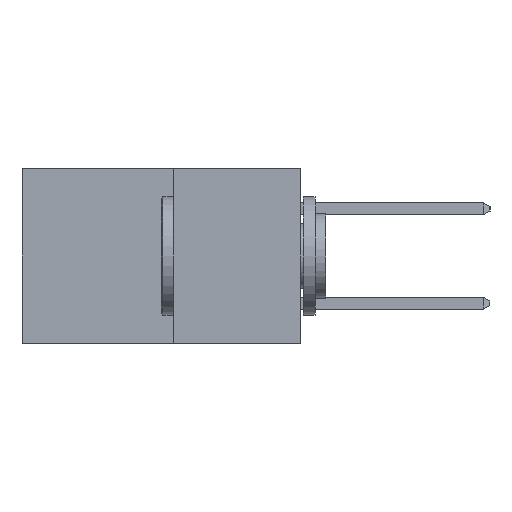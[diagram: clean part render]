
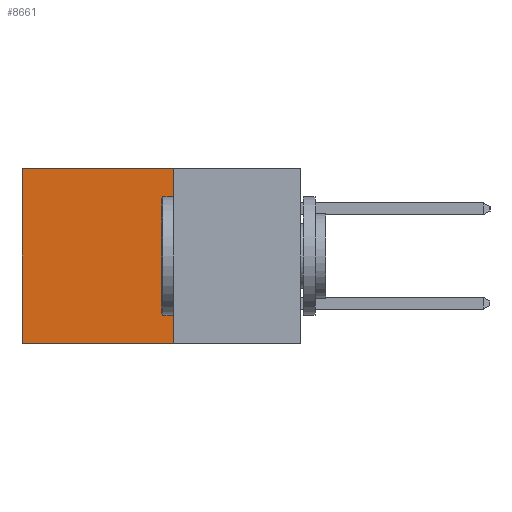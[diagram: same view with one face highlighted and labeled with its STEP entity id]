
A CAD part, left-side view. The second image highlights one B-rep face of the part: STEP entity #8661.
In plain terms, the highlighted planar face has unit normal (-1, 0, 0).
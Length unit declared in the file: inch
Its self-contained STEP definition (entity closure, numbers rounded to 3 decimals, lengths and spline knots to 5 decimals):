
#119 = CARTESIAN_POINT ( 'NONE',  ( 0.277, 0.59, -0.37 ) ) ;
#309 = LINE ( 'NONE', #3089, #3862 ) ;
#445 = LINE ( 'NONE', #697, #2233 ) ;
#697 = CARTESIAN_POINT ( 'NONE',  ( 0.277, 0.27, -0.37 ) ) ;
#1018 = EDGE_CURVE ( 'NONE', #4037, #9228, #309, .T. ) ;
#1445 = VECTOR ( 'NONE', #2529, 39.37008 ) ;
#1720 = CARTESIAN_POINT ( 'NONE',  ( 0.277, 0.27, 0. ) ) ;
#2233 = VECTOR ( 'NONE', #6638, 39.37008 ) ;
#2307 = EDGE_CURVE ( 'NONE', #4507, #9004, #8526, .T. ) ;
#2435 = PLANE ( 'NONE',  #4062 ) ;
#2528 = EDGE_CURVE ( 'NONE', #9228, #9004, #8627, .T. ) ;
#2529 = DIRECTION ( 'NONE',  ( 0., 1., 0. ) ) ;
#3036 = CARTESIAN_POINT ( 'NONE',  ( 0.277, 0.27, -0.37 ) ) ;
#3089 = CARTESIAN_POINT ( 'NONE',  ( 0.277, 0.27, 0. ) ) ;
#3189 = CARTESIAN_POINT ( 'NONE',  ( 0.277, 0.27, -0.37 ) ) ;
#3222 = DIRECTION ( 'NONE',  ( 0., 0., -1. ) ) ;
#3862 = VECTOR ( 'NONE', #6976, 39.37008 ) ;
#4037 = VERTEX_POINT ( 'NONE', #1720 ) ;
#4062 = AXIS2_PLACEMENT_3D ( 'NONE', #3189, #7493, #3222 ) ;
#4448 = ORIENTED_EDGE ( 'NONE', *, *, #1018, .T. ) ;
#4507 = VERTEX_POINT ( 'NONE', #3036 ) ;
#4889 = ORIENTED_EDGE ( 'NONE', *, *, #2307, .F. ) ;
#4900 = VECTOR ( 'NONE', #5539, 39.37008 ) ;
#5539 = DIRECTION ( 'NONE',  ( 0., 0., -1. ) ) ;
#5929 = ORIENTED_EDGE ( 'NONE', *, *, #2528, .T. ) ;
#6231 = CARTESIAN_POINT ( 'NONE',  ( 0.277, 0.27, -0.37 ) ) ;
#6290 = CARTESIAN_POINT ( 'NONE',  ( 0.277, 0.59, -0.37 ) ) ;
#6638 = DIRECTION ( 'NONE',  ( 0., 0., -1. ) ) ;
#6719 = EDGE_CURVE ( 'NONE', #4037, #4507, #445, .T. ) ;
#6793 = FACE_OUTER_BOUND ( 'NONE', #7451, .T. ) ;
#6976 = DIRECTION ( 'NONE',  ( 0., 1., 0. ) ) ;
#7343 = ORIENTED_EDGE ( 'NONE', *, *, #6719, .F. ) ;
#7451 = EDGE_LOOP ( 'NONE', ( #5929, #4889, #7343, #4448 ) ) ;
#7493 = DIRECTION ( 'NONE',  ( 1., 0., 0. ) ) ;
#7631 = CARTESIAN_POINT ( 'NONE',  ( 0.277, 0.59, 0. ) ) ;
#8526 = LINE ( 'NONE', #6231, #1445 ) ;
#8627 = LINE ( 'NONE', #6290, #4900 ) ;
#8661 = ADVANCED_FACE ( 'NONE', ( #6793 ), #2435, .F. ) ;
#9004 = VERTEX_POINT ( 'NONE', #119 ) ;
#9228 = VERTEX_POINT ( 'NONE', #7631 ) ;
